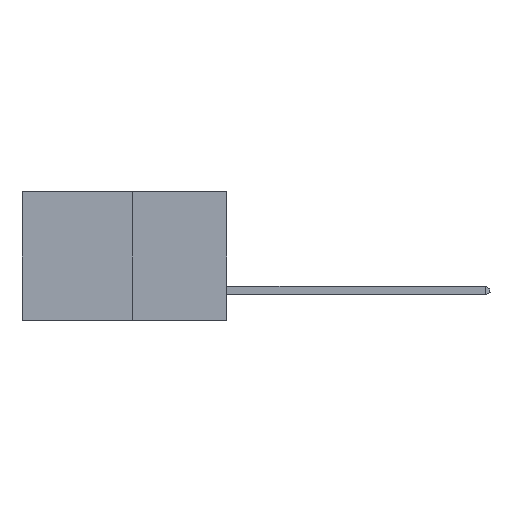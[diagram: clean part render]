
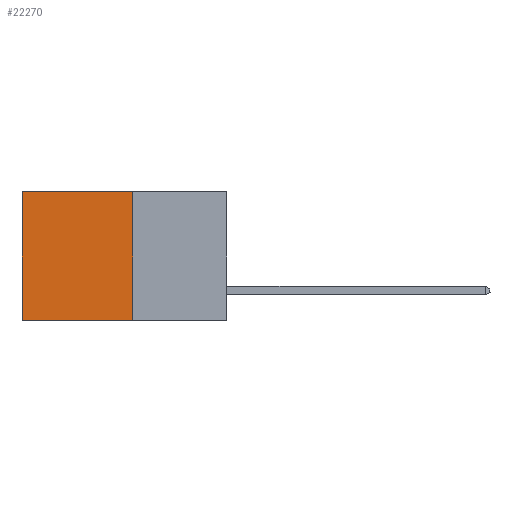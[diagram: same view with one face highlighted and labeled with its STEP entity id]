
A CAD part, left-side view. The second image highlights one B-rep face of the part: STEP entity #22270.
In plain terms, the highlighted planar face has unit normal (-1, 0, 0).
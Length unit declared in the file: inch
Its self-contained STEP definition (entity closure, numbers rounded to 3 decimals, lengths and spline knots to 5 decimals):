
#665 = EDGE_CURVE ( 'NONE', #22094, #11069, #18791, .T. ) ;
#1437 = CARTESIAN_POINT ( 'NONE',  ( 0.277, 0.59, 0. ) ) ;
#1873 = VECTOR ( 'NONE', #7575, 39.37008 ) ;
#2296 = EDGE_LOOP ( 'NONE', ( #11319, #21344, #20174, #15905 ) ) ;
#2689 = LINE ( 'NONE', #28183, #1873 ) ;
#3960 = CARTESIAN_POINT ( 'NONE',  ( 0.277, 0.27, -0.37 ) ) ;
#3984 = VERTEX_POINT ( 'NONE', #32376 ) ;
#4771 = PLANE ( 'NONE',  #22113 ) ;
#5231 = EDGE_CURVE ( 'NONE', #19622, #11069, #26133, .T. ) ;
#5908 = VECTOR ( 'NONE', #23431, 39.37008 ) ;
#7575 = DIRECTION ( 'NONE',  ( 0., 0., -1. ) ) ;
#9881 = VECTOR ( 'NONE', #19780, 39.37008 ) ;
#9965 = DIRECTION ( 'NONE',  ( 1., 0., 0. ) ) ;
#11069 = VERTEX_POINT ( 'NONE', #32766 ) ;
#11319 = ORIENTED_EDGE ( 'NONE', *, *, #665, .T. ) ;
#12104 = FACE_OUTER_BOUND ( 'NONE', #2296, .T. ) ;
#12434 = EDGE_CURVE ( 'NONE', #3984, #19622, #2689, .T. ) ;
#12495 = VECTOR ( 'NONE', #27118, 39.37008 ) ;
#15905 = ORIENTED_EDGE ( 'NONE', *, *, #15970, .T. ) ;
#15970 = EDGE_CURVE ( 'NONE', #3984, #22094, #16691, .T. ) ;
#16691 = LINE ( 'NONE', #32598, #9881 ) ;
#17596 = CARTESIAN_POINT ( 'NONE',  ( 0.277, 0.27, -0.37 ) ) ;
#18791 = LINE ( 'NONE', #31196, #5908 ) ;
#19622 = VERTEX_POINT ( 'NONE', #25175 ) ;
#19780 = DIRECTION ( 'NONE',  ( 0., 1., 0. ) ) ;
#20174 = ORIENTED_EDGE ( 'NONE', *, *, #12434, .F. ) ;
#21344 = ORIENTED_EDGE ( 'NONE', *, *, #5231, .F. ) ;
#22094 = VERTEX_POINT ( 'NONE', #1437 ) ;
#22113 = AXIS2_PLACEMENT_3D ( 'NONE', #17596, #9965, #27958 ) ;
#22270 = ADVANCED_FACE ( 'NONE', ( #12104 ), #4771, .F. ) ;
#23431 = DIRECTION ( 'NONE',  ( 0., 0., -1. ) ) ;
#25175 = CARTESIAN_POINT ( 'NONE',  ( 0.277, 0.27, -0.37 ) ) ;
#26133 = LINE ( 'NONE', #3960, #12495 ) ;
#27118 = DIRECTION ( 'NONE',  ( 0., 1., 0. ) ) ;
#27958 = DIRECTION ( 'NONE',  ( 0., 0., -1. ) ) ;
#28183 = CARTESIAN_POINT ( 'NONE',  ( 0.277, 0.27, -0.37 ) ) ;
#31196 = CARTESIAN_POINT ( 'NONE',  ( 0.277, 0.59, -0.37 ) ) ;
#32376 = CARTESIAN_POINT ( 'NONE',  ( 0.277, 0.27, 0. ) ) ;
#32598 = CARTESIAN_POINT ( 'NONE',  ( 0.277, 0.27, 0. ) ) ;
#32766 = CARTESIAN_POINT ( 'NONE',  ( 0.277, 0.59, -0.37 ) ) ;
